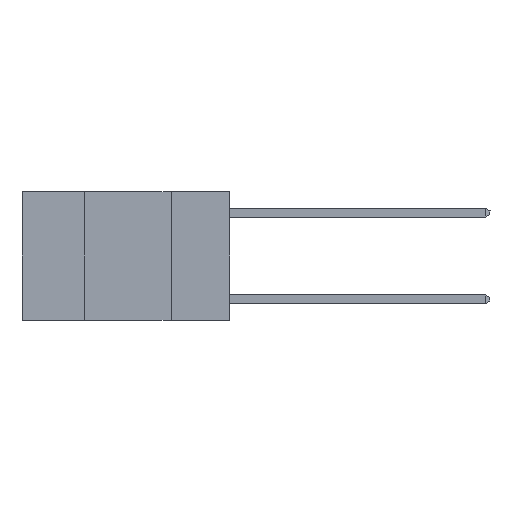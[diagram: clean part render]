
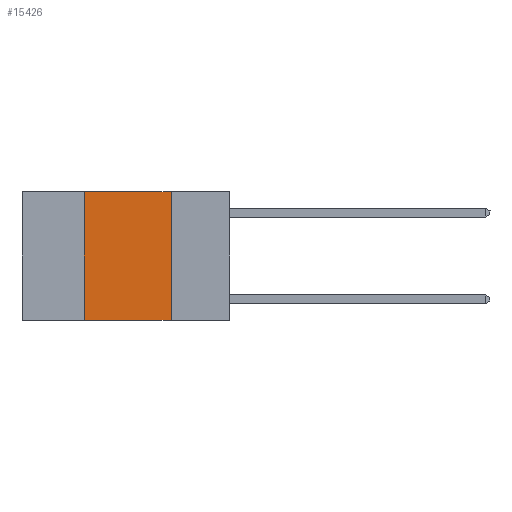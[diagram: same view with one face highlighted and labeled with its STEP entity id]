
A CAD part, left-side view. The second image highlights one B-rep face of the part: STEP entity #15426.
In plain terms, the highlighted planar face has unit normal (-1, 0, 0).
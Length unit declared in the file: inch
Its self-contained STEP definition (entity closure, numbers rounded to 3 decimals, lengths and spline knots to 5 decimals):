
#721 = CARTESIAN_POINT ( 'NONE',  ( 0., 0.42, 0. ) ) ;
#1014 = EDGE_CURVE ( 'NONE', #12639, #16020, #1690, .T. ) ;
#1159 = EDGE_CURVE ( 'NONE', #1594, #12639, #2787, .T. ) ;
#1594 = VERTEX_POINT ( 'NONE', #16167 ) ;
#1690 = LINE ( 'NONE', #13764, #15091 ) ;
#2191 = CARTESIAN_POINT ( 'NONE',  ( 0., 0.17, -0.37 ) ) ;
#2582 = LINE ( 'NONE', #721, #5808 ) ;
#2721 = CARTESIAN_POINT ( 'NONE',  ( 0., 0.17, 0. ) ) ;
#2760 = EDGE_CURVE ( 'NONE', #5029, #16020, #5381, .T. ) ;
#2787 = LINE ( 'NONE', #6143, #16521 ) ;
#3741 = DIRECTION ( 'NONE',  ( 1., 0., 0. ) ) ;
#5029 = VERTEX_POINT ( 'NONE', #5129 ) ;
#5129 = CARTESIAN_POINT ( 'NONE',  ( 0., 0.42, -0.37 ) ) ;
#5381 = LINE ( 'NONE', #9836, #15512 ) ;
#5808 = VECTOR ( 'NONE', #7550, 39.37008 ) ;
#6143 = CARTESIAN_POINT ( 'NONE',  ( 0., 0.6, 0. ) ) ;
#6414 = CARTESIAN_POINT ( 'NONE',  ( 0., 0.6, 0. ) ) ;
#6734 = ORIENTED_EDGE ( 'NONE', *, *, #16660, .F. ) ;
#7177 = DIRECTION ( 'NONE',  ( 0., 0., -1. ) ) ;
#7550 = DIRECTION ( 'NONE',  ( 0., 0., 1. ) ) ;
#7683 = FACE_OUTER_BOUND ( 'NONE', #17152, .T. ) ;
#9042 = PLANE ( 'NONE',  #9799 ) ;
#9799 = AXIS2_PLACEMENT_3D ( 'NONE', #6414, #3741, #13053 ) ;
#9822 = ORIENTED_EDGE ( 'NONE', *, *, #1159, .F. ) ;
#9836 = CARTESIAN_POINT ( 'NONE',  ( 0., 0.6, -0.37 ) ) ;
#11192 = DIRECTION ( 'NONE',  ( 0., -1., 0. ) ) ;
#12639 = VERTEX_POINT ( 'NONE', #2721 ) ;
#12742 = DIRECTION ( 'NONE',  ( 0., -1., 0. ) ) ;
#12938 = ORIENTED_EDGE ( 'NONE', *, *, #1014, .F. ) ;
#13053 = DIRECTION ( 'NONE',  ( 0., 0., -1. ) ) ;
#13764 = CARTESIAN_POINT ( 'NONE',  ( 0., 0.17, 0. ) ) ;
#15091 = VECTOR ( 'NONE', #7177, 39.37008 ) ;
#15426 = ADVANCED_FACE ( 'NONE', ( #7683 ), #9042, .F. ) ;
#15512 = VECTOR ( 'NONE', #11192, 39.37008 ) ;
#16020 = VERTEX_POINT ( 'NONE', #2191 ) ;
#16167 = CARTESIAN_POINT ( 'NONE',  ( 0., 0.42, 0. ) ) ;
#16521 = VECTOR ( 'NONE', #12742, 39.37008 ) ;
#16660 = EDGE_CURVE ( 'NONE', #5029, #1594, #2582, .T. ) ;
#17152 = EDGE_LOOP ( 'NONE', ( #12938, #9822, #6734, #17257 ) ) ;
#17257 = ORIENTED_EDGE ( 'NONE', *, *, #2760, .T. ) ;
